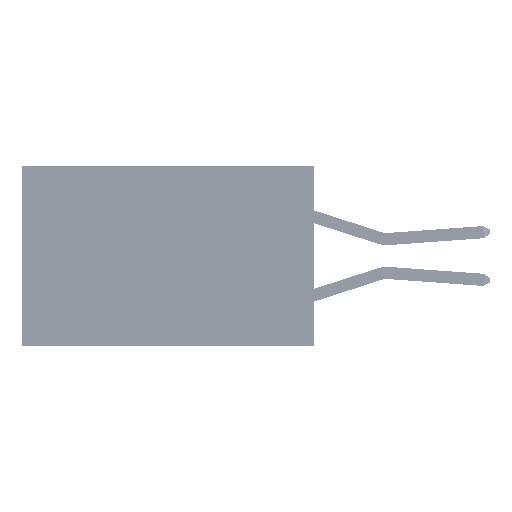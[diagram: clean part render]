
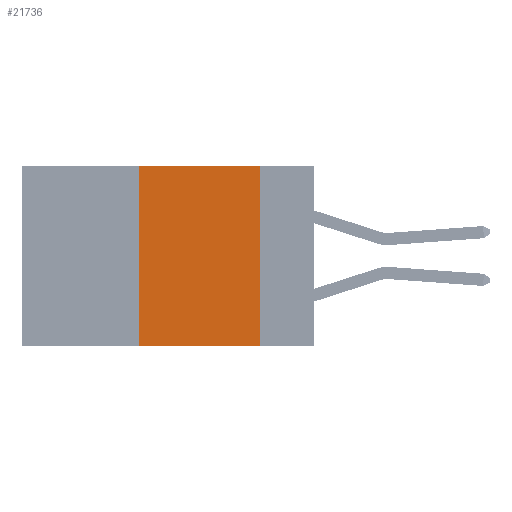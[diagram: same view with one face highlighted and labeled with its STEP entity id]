
A CAD part, left-side view. The second image highlights one B-rep face of the part: STEP entity #21736.
In plain terms, the highlighted planar face has unit normal (-1, 0, 0).
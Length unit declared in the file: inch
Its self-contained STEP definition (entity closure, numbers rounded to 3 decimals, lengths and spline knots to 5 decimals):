
#35 = ORIENTED_EDGE ( 'NONE', *, *, #23722, .T. ) ;
#1517 = VECTOR ( 'NONE', #14337, 39.37008 ) ;
#3287 = ORIENTED_EDGE ( 'NONE', *, *, #39102, .F. ) ;
#3923 = VERTEX_POINT ( 'NONE', #35904 ) ;
#4957 = CARTESIAN_POINT ( 'NONE',  ( 0., 0.36, -0.37 ) ) ;
#6118 = VECTOR ( 'NONE', #49454, 39.37008 ) ;
#6287 = ORIENTED_EDGE ( 'NONE', *, *, #28679, .F. ) ;
#6800 = VECTOR ( 'NONE', #41924, 39.37008 ) ;
#8387 = LINE ( 'NONE', #34383, #1517 ) ;
#8867 = CARTESIAN_POINT ( 'NONE',  ( 0., 0.6, -0.37 ) ) ;
#9304 = VERTEX_POINT ( 'NONE', #33136 ) ;
#9440 = AXIS2_PLACEMENT_3D ( 'NONE', #40537, #15931, #24235 ) ;
#9724 = CARTESIAN_POINT ( 'NONE',  ( 0., 0.6, 0. ) ) ;
#12391 = VERTEX_POINT ( 'NONE', #51369 ) ;
#13709 = LINE ( 'NONE', #8867, #6118 ) ;
#14337 = DIRECTION ( 'NONE',  ( 0., 0., 1. ) ) ;
#15770 = PLANE ( 'NONE',  #9440 ) ;
#15931 = DIRECTION ( 'NONE',  ( 1., 0., 0. ) ) ;
#16742 = CARTESIAN_POINT ( 'NONE',  ( 0., 0.11, 0. ) ) ;
#19348 = ORIENTED_EDGE ( 'NONE', *, *, #49351, .F. ) ;
#21736 = ADVANCED_FACE ( 'NONE', ( #32169 ), #15770, .F. ) ;
#23722 = EDGE_CURVE ( 'NONE', #33914, #3923, #13709, .T. ) ;
#24235 = DIRECTION ( 'NONE',  ( 0., 0., -1. ) ) ;
#27464 = LINE ( 'NONE', #16742, #38160 ) ;
#28679 = EDGE_CURVE ( 'NONE', #33914, #12391, #8387, .T. ) ;
#32169 = FACE_OUTER_BOUND ( 'NONE', #33935, .T. ) ;
#33136 = CARTESIAN_POINT ( 'NONE',  ( 0., 0.11, 0. ) ) ;
#33914 = VERTEX_POINT ( 'NONE', #4957 ) ;
#33935 = EDGE_LOOP ( 'NONE', ( #3287, #19348, #6287, #35 ) ) ;
#34383 = CARTESIAN_POINT ( 'NONE',  ( 0., 0.36, 0. ) ) ;
#35904 = CARTESIAN_POINT ( 'NONE',  ( 0., 0.11, -0.37 ) ) ;
#37152 = DIRECTION ( 'NONE',  ( 0., 0., -1. ) ) ;
#38160 = VECTOR ( 'NONE', #37152, 39.37008 ) ;
#38920 = LINE ( 'NONE', #9724, #6800 ) ;
#39102 = EDGE_CURVE ( 'NONE', #9304, #3923, #27464, .T. ) ;
#40537 = CARTESIAN_POINT ( 'NONE',  ( 0., 0.6, 0. ) ) ;
#41924 = DIRECTION ( 'NONE',  ( 0., -1., 0. ) ) ;
#49351 = EDGE_CURVE ( 'NONE', #12391, #9304, #38920, .T. ) ;
#49454 = DIRECTION ( 'NONE',  ( 0., -1., 0. ) ) ;
#51369 = CARTESIAN_POINT ( 'NONE',  ( 0., 0.36, 0. ) ) ;
